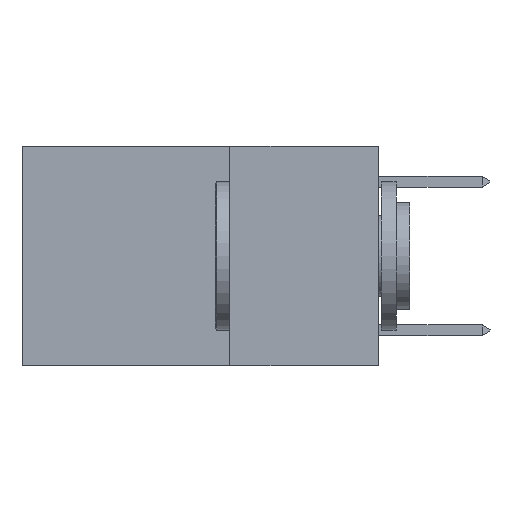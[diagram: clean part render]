
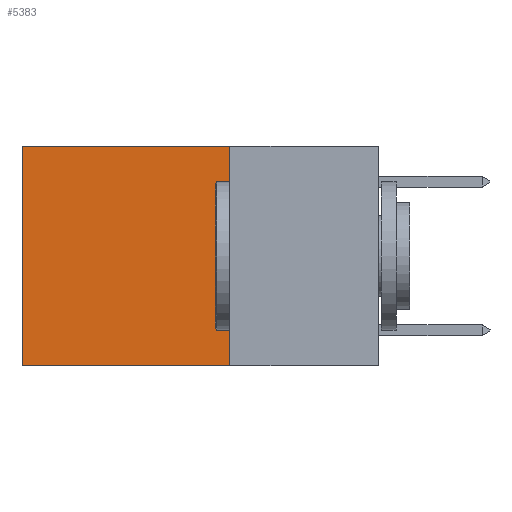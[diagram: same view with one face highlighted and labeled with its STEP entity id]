
A CAD part, left-side view. The second image highlights one B-rep face of the part: STEP entity #5383.
In plain terms, the highlighted planar face has unit normal (-1, 0, 0).
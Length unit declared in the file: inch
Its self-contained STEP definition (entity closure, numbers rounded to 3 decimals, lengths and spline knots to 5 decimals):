
#777 = VERTEX_POINT ( 'NONE', #27768 ) ;
#1021 = EDGE_LOOP ( 'NONE', ( #25164, #18793, #26233, #12310 ) ) ;
#2857 = VERTEX_POINT ( 'NONE', #26515 ) ;
#3244 = DIRECTION ( 'NONE',  ( 0., 0., -1. ) ) ;
#3715 = DIRECTION ( 'NONE',  ( 0., 1., 0. ) ) ;
#5383 = ADVANCED_FACE ( 'NONE', ( #6435 ), #20566, .F. ) ;
#5615 = CARTESIAN_POINT ( 'NONE',  ( 0.2625, 0.25, -0.37 ) ) ;
#6232 = VERTEX_POINT ( 'NONE', #24727 ) ;
#6435 = FACE_OUTER_BOUND ( 'NONE', #1021, .T. ) ;
#6711 = VECTOR ( 'NONE', #8059, 39.37008 ) ;
#8059 = DIRECTION ( 'NONE',  ( 0., 0., -1. ) ) ;
#8164 = CARTESIAN_POINT ( 'NONE',  ( 0.2625, 0.25, 0. ) ) ;
#8629 = EDGE_CURVE ( 'NONE', #777, #6232, #24595, .T. ) ;
#9754 = LINE ( 'NONE', #8164, #6711 ) ;
#10058 = LINE ( 'NONE', #24994, #21308 ) ;
#10993 = DIRECTION ( 'NONE',  ( 0., 0., -1. ) ) ;
#12310 = ORIENTED_EDGE ( 'NONE', *, *, #18821, .T. ) ;
#14150 = DIRECTION ( 'NONE',  ( 0., 1., 0. ) ) ;
#14878 = EDGE_CURVE ( 'NONE', #2857, #777, #9754, .T. ) ;
#16242 = VERTEX_POINT ( 'NONE', #21671 ) ;
#17750 = LINE ( 'NONE', #24040, #21489 ) ;
#18793 = ORIENTED_EDGE ( 'NONE', *, *, #8629, .F. ) ;
#18821 = EDGE_CURVE ( 'NONE', #2857, #16242, #10058, .T. ) ;
#20366 = CARTESIAN_POINT ( 'NONE',  ( 0.2625, 0.25, 0. ) ) ;
#20566 = PLANE ( 'NONE',  #26635 ) ;
#21308 = VECTOR ( 'NONE', #14150, 39.37008 ) ;
#21489 = VECTOR ( 'NONE', #10993, 39.37008 ) ;
#21671 = CARTESIAN_POINT ( 'NONE',  ( 0.2625, 0.6, 0. ) ) ;
#23575 = EDGE_CURVE ( 'NONE', #16242, #6232, #17750, .T. ) ;
#24006 = DIRECTION ( 'NONE',  ( 1., 0., 0. ) ) ;
#24040 = CARTESIAN_POINT ( 'NONE',  ( 0.2625, 0.6, 0. ) ) ;
#24595 = LINE ( 'NONE', #5615, #27324 ) ;
#24727 = CARTESIAN_POINT ( 'NONE',  ( 0.2625, 0.6, -0.37 ) ) ;
#24994 = CARTESIAN_POINT ( 'NONE',  ( 0.2625, 0.25, 0. ) ) ;
#25164 = ORIENTED_EDGE ( 'NONE', *, *, #23575, .T. ) ;
#26233 = ORIENTED_EDGE ( 'NONE', *, *, #14878, .F. ) ;
#26515 = CARTESIAN_POINT ( 'NONE',  ( 0.2625, 0.25, 0. ) ) ;
#26635 = AXIS2_PLACEMENT_3D ( 'NONE', #20366, #24006, #3244 ) ;
#27324 = VECTOR ( 'NONE', #3715, 39.37008 ) ;
#27768 = CARTESIAN_POINT ( 'NONE',  ( 0.2625, 0.25, -0.37 ) ) ;
